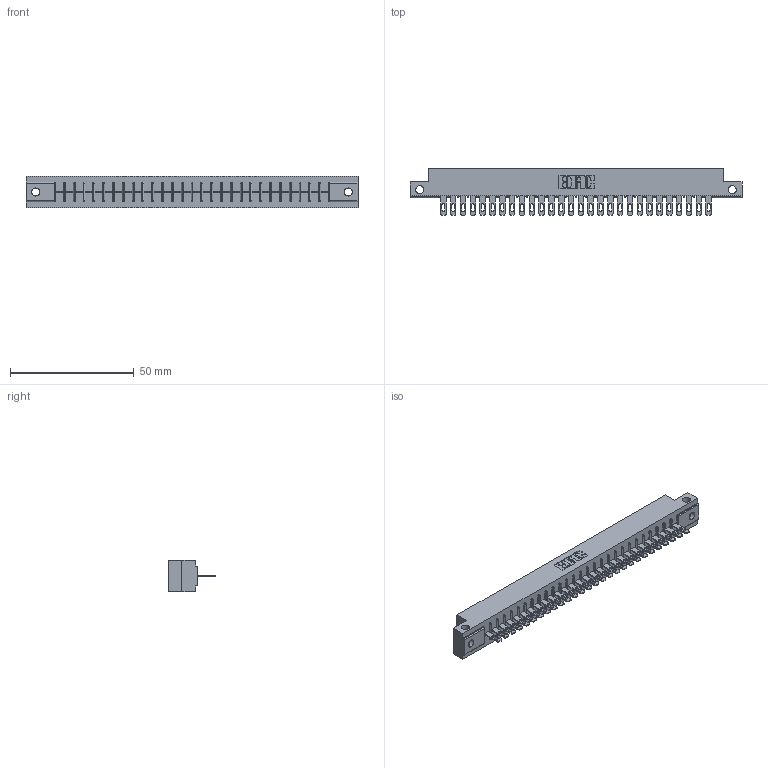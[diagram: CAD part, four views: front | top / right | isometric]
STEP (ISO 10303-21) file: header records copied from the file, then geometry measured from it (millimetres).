
FILE_DESCRIPTION (( 'STEP AP203' ), '1' );
FILE_NAME ('306-028-500-112.STEP', '2020-09-20T19:41:55', ( '' ), ( '' ), 'SwSTEP 2.0', 'SolidWorks 2020', '' );
FILE_SCHEMA (( 'CONFIG_CONTROL_DESIGN' ));
Length unit declared in the file: inch
Products named in the file (3): 306-290-001_100; 306 Part_.128 Dia; 306-028-500-112
Assembly tree (29 placements, depth 2):
  306-028-500-112
    306 Part_.128 Dia
    306-290-001_100  x28
Bounding box: 133.96 x 18.87 x 12.7 mm (x, y, z)
Volume: 14571.6 mm3; surface area: 15337.4 mm2
Topology: 29 solids, 29 shells, 2256 faces, 6372 edges, 4092 vertices
Faces by surface type: plane 1468, cylinder 676, sphere 112
Entity records: 28495 total; most frequent: CARTESIAN_POINT 4831, ORIENTED_EDGE 4744, DIRECTION 4704, EDGE_CURVE 2372, VECTOR 1830, LINE 1830, VERTEX_POINT 1500, AXIS2_PLACEMENT_3D 1437
